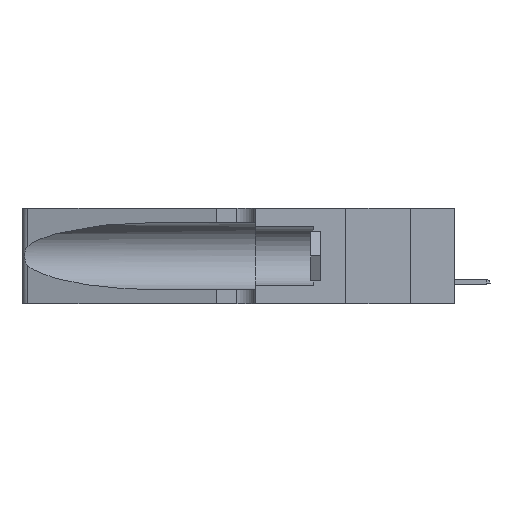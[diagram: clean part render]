
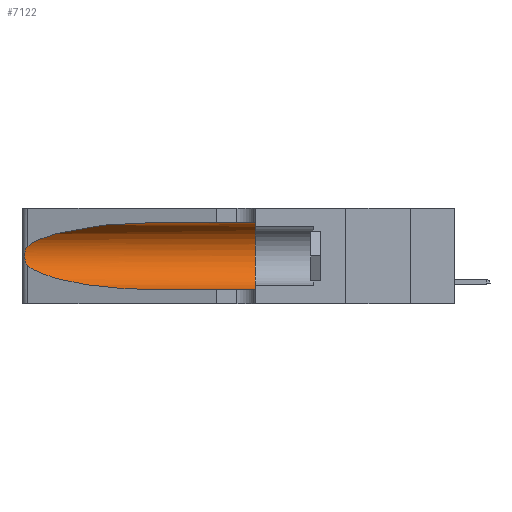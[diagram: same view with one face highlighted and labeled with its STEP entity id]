
A CAD part, left-side view. The second image highlights one B-rep face of the part: STEP entity #7122.
In plain terms, the highlighted cylindrical face has radius 3.308 mm (diameter 6.617 mm), a partial arc.
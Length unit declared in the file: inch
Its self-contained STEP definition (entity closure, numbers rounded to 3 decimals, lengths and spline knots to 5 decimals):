
#11 = ORIENTED_EDGE ( 'NONE', *, *, #4655, .T. ) ;
#126 = CIRCLE ( 'NONE', #4640, 0.13025 ) ;
#413 = VERTEX_POINT ( 'NONE', #14421 ) ;
#485 = DIRECTION ( 'NONE',  ( 0., 0., -1. ) ) ;
#636 = CARTESIAN_POINT ( 'NONE',  ( 0.25639, 1.23186, 0.15144 ) ) ;
#650 = EDGE_CURVE ( 'NONE', #14708, #18388, #15819, .T. ) ;
#1048 = EDGE_CURVE ( 'NONE', #413, #1622, #126, .T. ) ;
#1105 = VECTOR ( 'NONE', #9861, 39.37008 ) ;
#1271 = CARTESIAN_POINT ( 'NONE',  ( 0.25487, 1.22718, 0.14631 ) ) ;
#1358 = CARTESIAN_POINT ( 'NONE',  ( 0.2373, 1.15595, 0.08982 ) ) ;
#1436 = CARTESIAN_POINT ( 'NONE',  ( 0.1305, 0.72297, 0.31525 ) ) ;
#1604 = EDGE_CURVE ( 'NONE', #4419, #413, #13115, .T. ) ;
#1622 = VERTEX_POINT ( 'NONE', #7565 ) ;
#1727 = ORIENTED_EDGE ( 'NONE', *, *, #650, .T. ) ;
#1865 = CARTESIAN_POINT ( 'NONE',  ( 0.1305, 1.61858, 0.31525 ) ) ;
#2048 = CARTESIAN_POINT ( 'NONE',  ( 0.26075, 1.23896, 0.19203 ) ) ;
#2091 = DIRECTION ( 'NONE',  ( 0., -1., 0. ) ) ;
#2330 = CARTESIAN_POINT ( 'NONE',  ( 0.26075, 1.23896, 0.178 ) ) ;
#2477 = CARTESIAN_POINT ( 'NONE',  ( 0.1305, 0.35, 0.185 ) ) ;
#2761 = ORIENTED_EDGE ( 'NONE', *, *, #8725, .T. ) ;
#3218 = CARTESIAN_POINT ( 'NONE',  ( 0.1305, 1.61858, 0.185 ) ) ;
#3267 = B_SPLINE_CURVE_WITH_KNOTS ( 'NONE', 3,
 ( #3644, #16502, #3726, #16311, #9371, #15078, #2048, #2330, #3464, #10856, #13761, #636, #10672, #9182 ),
 .UNSPECIFIED., .F., .F.,
 ( 4, 2, 2, 2, 2, 2, 4 ),
 ( 0., 0.00027, 0.00053, 0.00107, 0.0016, 0.00187, 0.00214 ),
 .UNSPECIFIED. ) ;
#3421 = VECTOR ( 'NONE', #15918, 39.37008 ) ;
#3464 = CARTESIAN_POINT ( 'NONE',  ( 0.26017, 1.23833, 0.17102 ) ) ;
#3583 = ORIENTED_EDGE ( 'NONE', *, *, #15110, .T. ) ;
#3644 = CARTESIAN_POINT ( 'NONE',  ( 0.25487, 1.22718, 0.22369 ) ) ;
#3726 = CARTESIAN_POINT ( 'NONE',  ( 0.25639, 1.23184, 0.21858 ) ) ;
#4147 = DIRECTION ( 'NONE',  ( 0., 1., 0. ) ) ;
#4419 = VERTEX_POINT ( 'NONE', #14429 ) ;
#4640 = AXIS2_PLACEMENT_3D ( 'NONE', #2477, #4147, #8186 ) ;
#4655 = EDGE_CURVE ( 'NONE', #6984, #14708, #3267, .T. ) ;
#4883 = ORIENTED_EDGE ( 'NONE', *, *, #1048, .F. ) ;
#6671 = CARTESIAN_POINT ( 'NONE',  ( 0.1305, 0.72297, 0.05475 ) ) ;
#6984 = VERTEX_POINT ( 'NONE', #17371 ) ;
#7122 = ADVANCED_FACE ( 'NONE', ( #9025 ), #7700, .F. ) ;
#7565 = CARTESIAN_POINT ( 'NONE',  ( 0.1305, 0.35, 0.05475 ) ) ;
#7700 = CYLINDRICAL_SURFACE ( 'NONE', #13630, 0.13025 ) ;
#8186 = DIRECTION ( 'NONE',  ( 0., 0., 1. ) ) ;
#8725 = EDGE_CURVE ( 'NONE', #18388, #1622, #15564, .T. ) ;
#8842 = CARTESIAN_POINT ( 'NONE',  ( 0.2373, 1.15595, 0.28018 ) ) ;
#9025 = FACE_OUTER_BOUND ( 'NONE', #13646, .T. ) ;
#9182 = CARTESIAN_POINT ( 'NONE',  ( 0.25487, 1.22718, 0.14631 ) ) ;
#9371 = CARTESIAN_POINT ( 'NONE',  ( 0.25854, 1.2359, 0.20912 ) ) ;
#9861 = DIRECTION ( 'NONE',  ( 0., -1., 0. ) ) ;
#9950 = CARTESIAN_POINT ( 'NONE',  ( 0.1305, 1.61858, 0.05475 ) ) ;
#10039 = CARTESIAN_POINT ( 'NONE',  ( 0.25487, 1.22718, 0.14631 ) ) ;
#10672 = CARTESIAN_POINT ( 'NONE',  ( 0.25555, 1.22993, 0.14849 ) ) ;
#10856 = CARTESIAN_POINT ( 'NONE',  ( 0.25856, 1.23593, 0.16098 ) ) ;
#12752 = ORIENTED_EDGE ( 'NONE', *, *, #1604, .F. ) ;
#13115 = LINE ( 'NONE', #1865, #3421 ) ;
#13630 = AXIS2_PLACEMENT_3D ( 'NONE', #3218, #2091, #485 ) ;
#13646 = EDGE_LOOP ( 'NONE', ( #3583, #11, #1727, #2761, #4883, #12752 ) ) ;
#13761 = CARTESIAN_POINT ( 'NONE',  ( 0.25789, 1.23486, 0.15765 ) ) ;
#14299 = CARTESIAN_POINT ( 'NONE',  ( 0.1305, 0.72297, 0.05475 ) ) ;
#14421 = CARTESIAN_POINT ( 'NONE',  ( 0.1305, 0.35, 0.31525 ) ) ;
#14429 = CARTESIAN_POINT ( 'NONE',  ( 0.1305, 0.72297, 0.31525 ) ) ;
#14708 = VERTEX_POINT ( 'NONE', #10039 ) ;
#15078 = CARTESIAN_POINT ( 'NONE',  ( 0.26018, 1.23835, 0.19895 ) ) ;
#15110 = EDGE_CURVE ( 'NONE', #4419, #6984, #17626, .T. ) ;
#15564 = LINE ( 'NONE', #9950, #1105 ) ;
#15819 =( BOUNDED_CURVE ( )  B_SPLINE_CURVE ( 3, ( #1271, #1358, #16848, #14299 ),
 .UNSPECIFIED., .F., .F. ) 
 B_SPLINE_CURVE_WITH_KNOTS ( ( 4, 4 ),
 ( 3.44316, 4.71239 ),
 .UNSPECIFIED. ) 
 CURVE ( )  GEOMETRIC_REPRESENTATION_ITEM ( )  RATIONAL_B_SPLINE_CURVE ( ( 1., 0.87, 0.87, 1. ) ) 
 REPRESENTATION_ITEM ( '' )  );
#15918 = DIRECTION ( 'NONE',  ( 0., -1., 0. ) ) ;
#16311 = CARTESIAN_POINT ( 'NONE',  ( 0.25787, 1.23484, 0.2124 ) ) ;
#16502 = CARTESIAN_POINT ( 'NONE',  ( 0.25555, 1.22994, 0.2215 ) ) ;
#16848 = CARTESIAN_POINT ( 'NONE',  ( 0.18966, 0.96281, 0.05475 ) ) ;
#17371 = CARTESIAN_POINT ( 'NONE',  ( 0.25487, 1.22718, 0.22369 ) ) ;
#17376 = CARTESIAN_POINT ( 'NONE',  ( 0.18966, 0.96281, 0.31525 ) ) ;
#17474 = CARTESIAN_POINT ( 'NONE',  ( 0.25487, 1.22718, 0.22369 ) ) ;
#17626 =( BOUNDED_CURVE ( )  B_SPLINE_CURVE ( 3, ( #1436, #17376, #8842, #17474 ),
 .UNSPECIFIED., .F., .T. ) 
 B_SPLINE_CURVE_WITH_KNOTS ( ( 4, 4 ),
 ( 1.5708, 2.84003 ),
 .UNSPECIFIED. ) 
 CURVE ( )  GEOMETRIC_REPRESENTATION_ITEM ( )  RATIONAL_B_SPLINE_CURVE ( ( 1., 0.87, 0.87, 1. ) ) 
 REPRESENTATION_ITEM ( '' )  );
#18388 = VERTEX_POINT ( 'NONE', #6671 ) ;
